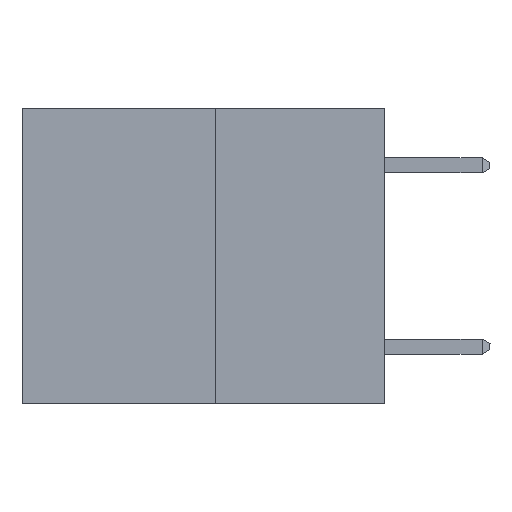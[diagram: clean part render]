
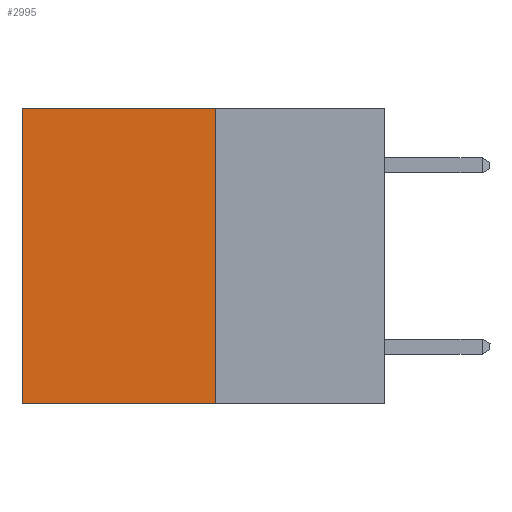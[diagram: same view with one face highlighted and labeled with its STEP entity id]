
A CAD part, left-side view. The second image highlights one B-rep face of the part: STEP entity #2995.
In plain terms, the highlighted planar face has unit normal (-1, 0, 0).
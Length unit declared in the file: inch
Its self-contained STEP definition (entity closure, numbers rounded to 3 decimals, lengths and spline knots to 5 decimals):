
#1917 = CARTESIAN_POINT ( 'NONE',  ( 0.3165, 0.28, -0.49 ) ) ;
#1955 = DIRECTION ( 'NONE',  ( 0., 1., 0. ) ) ;
#2284 = VERTEX_POINT ( 'NONE', #13029 ) ;
#2635 = EDGE_CURVE ( 'NONE', #9430, #14003, #4822, .T. ) ;
#2818 = EDGE_CURVE ( 'NONE', #2284, #9430, #11895, .T. ) ;
#2995 = ADVANCED_FACE ( 'NONE', ( #4755 ), #17557, .F. ) ;
#3083 = ORIENTED_EDGE ( 'NONE', *, *, #15099, .F. ) ;
#3249 = DIRECTION ( 'NONE',  ( 0., 1., 0. ) ) ;
#3274 = CARTESIAN_POINT ( 'NONE',  ( 0.3165, 0.6, -0.49 ) ) ;
#3294 = ORIENTED_EDGE ( 'NONE', *, *, #2635, .T. ) ;
#4335 = ORIENTED_EDGE ( 'NONE', *, *, #14670, .F. ) ;
#4490 = CARTESIAN_POINT ( 'NONE',  ( 0.3165, 0.6, 0. ) ) ;
#4755 = FACE_OUTER_BOUND ( 'NONE', #11529, .T. ) ;
#4822 = LINE ( 'NONE', #7050, #18783 ) ;
#4973 = DIRECTION ( 'NONE',  ( 0., 0., -1. ) ) ;
#6907 = ORIENTED_EDGE ( 'NONE', *, *, #2818, .T. ) ;
#7050 = CARTESIAN_POINT ( 'NONE',  ( 0.3165, 0.6, -0.49 ) ) ;
#7472 = CARTESIAN_POINT ( 'NONE',  ( 0.3165, 0.28, -0.49 ) ) ;
#8542 = VERTEX_POINT ( 'NONE', #7472 ) ;
#9430 = VERTEX_POINT ( 'NONE', #4490 ) ;
#10105 = AXIS2_PLACEMENT_3D ( 'NONE', #19182, #12954, #16036 ) ;
#11529 = EDGE_LOOP ( 'NONE', ( #3294, #4335, #3083, #6907 ) ) ;
#11725 = VECTOR ( 'NONE', #3249, 39.37008 ) ;
#11895 = LINE ( 'NONE', #16631, #19450 ) ;
#12954 = DIRECTION ( 'NONE',  ( 1., 0., 0. ) ) ;
#13029 = CARTESIAN_POINT ( 'NONE',  ( 0.3165, 0.28, 0. ) ) ;
#14003 = VERTEX_POINT ( 'NONE', #3274 ) ;
#14670 = EDGE_CURVE ( 'NONE', #8542, #14003, #15966, .T. ) ;
#15099 = EDGE_CURVE ( 'NONE', #2284, #8542, #17558, .T. ) ;
#15966 = LINE ( 'NONE', #19378, #11725 ) ;
#16036 = DIRECTION ( 'NONE',  ( 0., 0., -1. ) ) ;
#16631 = CARTESIAN_POINT ( 'NONE',  ( 0.3165, 0.28, 0. ) ) ;
#17307 = VECTOR ( 'NONE', #4973, 39.37008 ) ;
#17557 = PLANE ( 'NONE',  #10105 ) ;
#17558 = LINE ( 'NONE', #1917, #17307 ) ;
#18783 = VECTOR ( 'NONE', #19831, 39.37008 ) ;
#19182 = CARTESIAN_POINT ( 'NONE',  ( 0.3165, 0.28, -0.49 ) ) ;
#19378 = CARTESIAN_POINT ( 'NONE',  ( 0.3165, 0.28, -0.49 ) ) ;
#19450 = VECTOR ( 'NONE', #1955, 39.37008 ) ;
#19831 = DIRECTION ( 'NONE',  ( 0., 0., -1. ) ) ;
